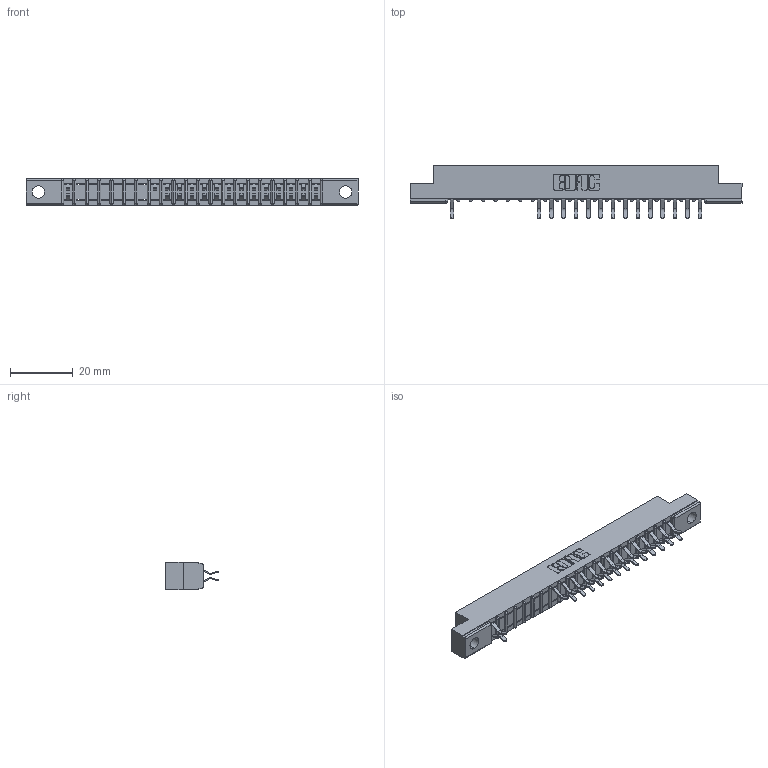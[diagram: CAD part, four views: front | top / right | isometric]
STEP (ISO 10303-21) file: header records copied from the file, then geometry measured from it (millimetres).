
FILE_DESCRIPTION (( 'STEP AP203' ), '1' );
FILE_NAME ('307-042-556-204.STEP', '2018-08-05T18:29:37', ( '' ), ( '' ), 'SwSTEP 2.0', 'SolidWorks 2016', '' );
FILE_SCHEMA (( 'CONFIG_CONTROL_DESIGN' ));
Length unit declared in the file: inch
Products named in the file (3): 307 Part_.156 Dia Mounting Holes; 307-290-001_556; 307-042-556-204
Assembly tree (30 placements, depth 2):
  307-042-556-204
    307 Part_.156 Dia Mounting Holes
    307-290-001_556  x29
Bounding box: 106.22 x 16.97 x 8.71 mm (x, y, z)
Volume: 6668.7 mm3; surface area: 10591.9 mm2
Topology: 30 solids, 30 shells, 1734 faces, 4893 edges, 3162 vertices
Faces by surface type: plane 1119, cylinder 571, sphere 44
Entity records: 21370 total; most frequent: CARTESIAN_POINT 3562, ORIENTED_EDGE 3538, DIRECTION 3477, EDGE_CURVE 1769, LINE 1355, VECTOR 1355, VERTEX_POINT 1146, AXIS2_PLACEMENT_3D 1061
